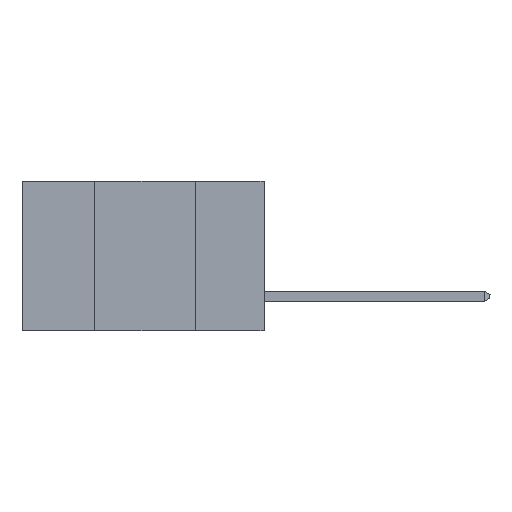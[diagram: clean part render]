
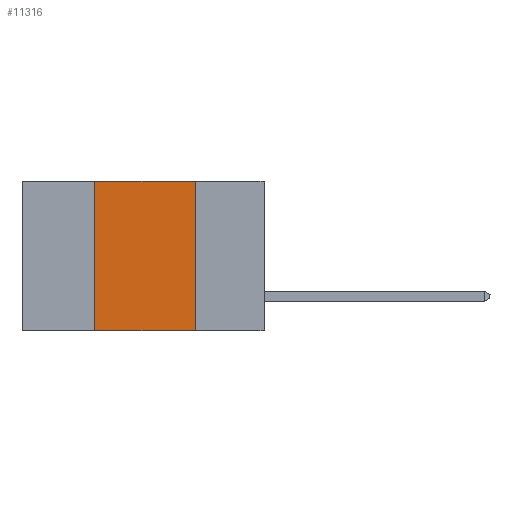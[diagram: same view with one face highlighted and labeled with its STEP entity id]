
A CAD part, left-side view. The second image highlights one B-rep face of the part: STEP entity #11316.
In plain terms, the highlighted planar face has unit normal (-1, 0, 0).
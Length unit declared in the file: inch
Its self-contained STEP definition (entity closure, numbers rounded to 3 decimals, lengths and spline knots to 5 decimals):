
#655 = LINE ( 'NONE', #6432, #16111 ) ;
#953 = VERTEX_POINT ( 'NONE', #3439 ) ;
#1380 = DIRECTION ( 'NONE',  ( 0., 0., -1. ) ) ;
#2374 = ORIENTED_EDGE ( 'NONE', *, *, #17681, .F. ) ;
#2950 = DIRECTION ( 'NONE',  ( 0., 0., 1. ) ) ;
#3060 = VECTOR ( 'NONE', #1380, 39.37008 ) ;
#3382 = VERTEX_POINT ( 'NONE', #9144 ) ;
#3439 = CARTESIAN_POINT ( 'NONE',  ( 0., 0.42, 0. ) ) ;
#3962 = ORIENTED_EDGE ( 'NONE', *, *, #17982, .F. ) ;
#5003 = CARTESIAN_POINT ( 'NONE',  ( 0., 0.6, -0.37 ) ) ;
#5194 = EDGE_LOOP ( 'NONE', ( #3962, #5865, #2374, #7052 ) ) ;
#5706 = EDGE_CURVE ( 'NONE', #953, #8084, #655, .T. ) ;
#5865 = ORIENTED_EDGE ( 'NONE', *, *, #5706, .F. ) ;
#6303 = LINE ( 'NONE', #5003, #11557 ) ;
#6432 = CARTESIAN_POINT ( 'NONE',  ( 0., 0.6, 0. ) ) ;
#7052 = ORIENTED_EDGE ( 'NONE', *, *, #13400, .T. ) ;
#8082 = LINE ( 'NONE', #17988, #3060 ) ;
#8084 = VERTEX_POINT ( 'NONE', #8316 ) ;
#8316 = CARTESIAN_POINT ( 'NONE',  ( 0., 0.17, 0. ) ) ;
#8795 = DIRECTION ( 'NONE',  ( 1., 0., 0. ) ) ;
#9144 = CARTESIAN_POINT ( 'NONE',  ( 0., 0.17, -0.37 ) ) ;
#9844 = CARTESIAN_POINT ( 'NONE',  ( 0., 0.42, -0.37 ) ) ;
#9998 = PLANE ( 'NONE',  #14766 ) ;
#11316 = ADVANCED_FACE ( 'NONE', ( #12837 ), #9998, .F. ) ;
#11557 = VECTOR ( 'NONE', #14638, 39.37008 ) ;
#11866 = DIRECTION ( 'NONE',  ( 0., -1., 0. ) ) ;
#12447 = VECTOR ( 'NONE', #2950, 39.37008 ) ;
#12686 = CARTESIAN_POINT ( 'NONE',  ( 0., 0.42, -0.37 ) ) ;
#12837 = FACE_OUTER_BOUND ( 'NONE', #5194, .T. ) ;
#13400 = EDGE_CURVE ( 'NONE', #14122, #3382, #6303, .T. ) ;
#14024 = DIRECTION ( 'NONE',  ( 0., 0., -1. ) ) ;
#14122 = VERTEX_POINT ( 'NONE', #9844 ) ;
#14638 = DIRECTION ( 'NONE',  ( 0., -1., 0. ) ) ;
#14766 = AXIS2_PLACEMENT_3D ( 'NONE', #15687, #8795, #14024 ) ;
#15687 = CARTESIAN_POINT ( 'NONE',  ( 0., 0.6, 0. ) ) ;
#16111 = VECTOR ( 'NONE', #11866, 39.37008 ) ;
#17179 = LINE ( 'NONE', #12686, #12447 ) ;
#17681 = EDGE_CURVE ( 'NONE', #14122, #953, #17179, .T. ) ;
#17982 = EDGE_CURVE ( 'NONE', #8084, #3382, #8082, .T. ) ;
#17988 = CARTESIAN_POINT ( 'NONE',  ( 0., 0.17, -0.37 ) ) ;
